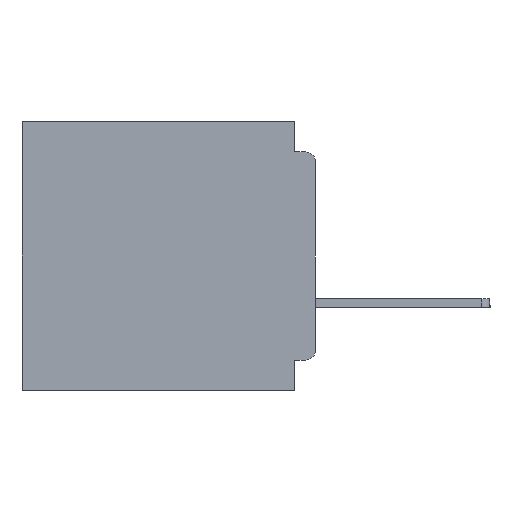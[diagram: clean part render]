
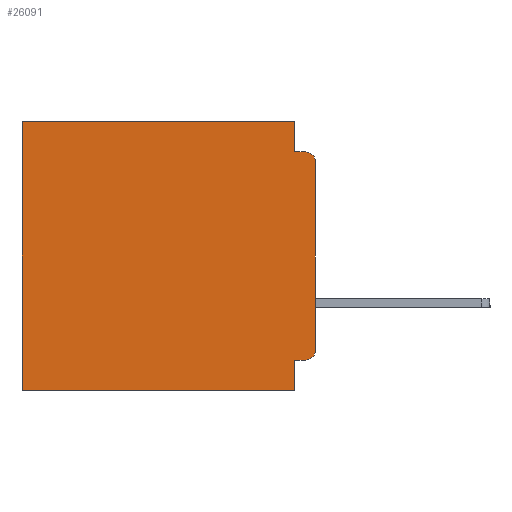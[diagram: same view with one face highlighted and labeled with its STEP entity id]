
A CAD part, left-side view. The second image highlights one B-rep face of the part: STEP entity #26091.
In plain terms, the highlighted planar face has unit normal (-1, 0, 0).
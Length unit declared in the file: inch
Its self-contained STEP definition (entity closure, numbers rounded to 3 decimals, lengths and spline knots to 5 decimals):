
#51 = DIRECTION ( 'NONE',  ( -1., 0., 0. ) ) ;
#653 = CARTESIAN_POINT ( 'NONE',  ( 0.3, 0., -0.34 ) ) ;
#697 = EDGE_CURVE ( 'NONE', #22691, #24776, #6762, .T. ) ;
#934 = EDGE_CURVE ( 'NONE', #24162, #24214, #21215, .T. ) ;
#1195 = VECTOR ( 'NONE', #26522, 39.37008 ) ;
#1617 = ORIENTED_EDGE ( 'NONE', *, *, #15779, .T. ) ;
#2592 = VERTEX_POINT ( 'NONE', #31737 ) ;
#3250 = CARTESIAN_POINT ( 'NONE',  ( 0.3, 0., -0.06 ) ) ;
#3530 = DIRECTION ( 'NONE',  ( 0., 0., -1. ) ) ;
#3794 = LINE ( 'NONE', #26457, #24612 ) ;
#4449 = VERTEX_POINT ( 'NONE', #22571 ) ;
#4848 = CARTESIAN_POINT ( 'NONE',  ( 0.3, 0.031, 0. ) ) ;
#5273 = VECTOR ( 'NONE', #8949, 39.37008 ) ;
#6329 = PLANE ( 'NONE',  #8413 ) ;
#6762 = LINE ( 'NONE', #13682, #28428 ) ;
#6907 = EDGE_CURVE ( 'NONE', #15076, #2592, #25308, .T. ) ;
#6944 = DIRECTION ( 'NONE',  ( 0., 0., -1. ) ) ;
#7821 = VECTOR ( 'NONE', #6944, 39.37008 ) ;
#8090 = CARTESIAN_POINT ( 'NONE',  ( 0.3, 0.015, -0.06 ) ) ;
#8413 = AXIS2_PLACEMENT_3D ( 'NONE', #26077, #12065, #31783 ) ;
#8621 = CARTESIAN_POINT ( 'NONE',  ( 0.3, 0., -0.4 ) ) ;
#8702 = LINE ( 'NONE', #23894, #7821 ) ;
#8949 = DIRECTION ( 'NONE',  ( 0., 0., -1. ) ) ;
#9824 = EDGE_CURVE ( 'NONE', #32559, #15076, #35727, .T. ) ;
#9935 = EDGE_CURVE ( 'NONE', #4449, #2592, #23817, .T. ) ;
#10116 = VECTOR ( 'NONE', #22009, 39.37008 ) ;
#10307 = VECTOR ( 'NONE', #26129, 39.37008 ) ;
#10469 = AXIS2_PLACEMENT_3D ( 'NONE', #8090, #27848, #10963 ) ;
#10963 = DIRECTION ( 'NONE',  ( 0., 0., -1. ) ) ;
#12027 = CARTESIAN_POINT ( 'NONE',  ( 0.3, 0.031, -0.4 ) ) ;
#12065 = DIRECTION ( 'NONE',  ( 1., 0., 0. ) ) ;
#12370 = VECTOR ( 'NONE', #3530, 39.37008 ) ;
#13682 = CARTESIAN_POINT ( 'NONE',  ( 0.3, 0., -0.045 ) ) ;
#14464 = CIRCLE ( 'NONE', #31461, 0.015 ) ;
#14805 = DIRECTION ( 'NONE',  ( 0., -1., 0. ) ) ;
#14817 = EDGE_CURVE ( 'NONE', #35808, #4449, #3794, .T. ) ;
#14842 = EDGE_CURVE ( 'NONE', #35808, #22691, #8702, .T. ) ;
#15076 = VERTEX_POINT ( 'NONE', #33397 ) ;
#15779 = EDGE_CURVE ( 'NONE', #23216, #24214, #14464, .T. ) ;
#17085 = CARTESIAN_POINT ( 'NONE',  ( 0.3, 0.015, -0.34 ) ) ;
#17675 = LINE ( 'NONE', #36063, #10116 ) ;
#18830 = EDGE_CURVE ( 'NONE', #24162, #24776, #29590, .T. ) ;
#19890 = DIRECTION ( 'NONE',  ( 0., 0., -1. ) ) ;
#21215 = LINE ( 'NONE', #8621, #5273 ) ;
#22009 = DIRECTION ( 'NONE',  ( 0., 1., 0. ) ) ;
#22571 = CARTESIAN_POINT ( 'NONE',  ( 0.3, 0.437, 0. ) ) ;
#22691 = VERTEX_POINT ( 'NONE', #30205 ) ;
#23216 = VERTEX_POINT ( 'NONE', #35714 ) ;
#23716 = CARTESIAN_POINT ( 'NONE',  ( 0.3, 0.437, -0.4 ) ) ;
#23817 = LINE ( 'NONE', #23716, #1195 ) ;
#23894 = CARTESIAN_POINT ( 'NONE',  ( 0.3, 0.031, 0. ) ) ;
#23969 = FACE_OUTER_BOUND ( 'NONE', #33503, .T. ) ;
#24162 = VERTEX_POINT ( 'NONE', #3250 ) ;
#24214 = VERTEX_POINT ( 'NONE', #653 ) ;
#24612 = VECTOR ( 'NONE', #35001, 39.37008 ) ;
#24776 = VERTEX_POINT ( 'NONE', #28713 ) ;
#25308 = LINE ( 'NONE', #28987, #10307 ) ;
#26077 = CARTESIAN_POINT ( 'NONE',  ( 0.3, 0., -0.4 ) ) ;
#26091 = ADVANCED_FACE ( 'NONE', ( #23969 ), #6329, .F. ) ;
#26129 = DIRECTION ( 'NONE',  ( 0., 1., 0. ) ) ;
#26457 = CARTESIAN_POINT ( 'NONE',  ( 0.3, 0., 0. ) ) ;
#26522 = DIRECTION ( 'NONE',  ( 0., 0., -1. ) ) ;
#27848 = DIRECTION ( 'NONE',  ( -1., 0., 0. ) ) ;
#28428 = VECTOR ( 'NONE', #14805, 39.37008 ) ;
#28656 = EDGE_CURVE ( 'NONE', #23216, #32559, #17675, .T. ) ;
#28713 = CARTESIAN_POINT ( 'NONE',  ( 0.3, 0.015, -0.045 ) ) ;
#28987 = CARTESIAN_POINT ( 'NONE',  ( 0.3, 0., -0.4 ) ) ;
#29137 = ORIENTED_EDGE ( 'NONE', *, *, #9935, .T. ) ;
#29404 = ORIENTED_EDGE ( 'NONE', *, *, #14817, .T. ) ;
#29590 = CIRCLE ( 'NONE', #10469, 0.015 ) ;
#30137 = ORIENTED_EDGE ( 'NONE', *, *, #14842, .F. ) ;
#30205 = CARTESIAN_POINT ( 'NONE',  ( 0.3, 0.031, -0.045 ) ) ;
#30388 = CARTESIAN_POINT ( 'NONE',  ( 0.3, 0.031, -0.355 ) ) ;
#30987 = ORIENTED_EDGE ( 'NONE', *, *, #697, .F. ) ;
#31461 = AXIS2_PLACEMENT_3D ( 'NONE', #17085, #51, #19890 ) ;
#31523 = ORIENTED_EDGE ( 'NONE', *, *, #18830, .T. ) ;
#31737 = CARTESIAN_POINT ( 'NONE',  ( 0.3, 0.437, -0.4 ) ) ;
#31783 = DIRECTION ( 'NONE',  ( 0., 0., -1. ) ) ;
#32193 = ORIENTED_EDGE ( 'NONE', *, *, #934, .F. ) ;
#32559 = VERTEX_POINT ( 'NONE', #30388 ) ;
#33397 = CARTESIAN_POINT ( 'NONE',  ( 0.3, 0.031, -0.4 ) ) ;
#33503 = EDGE_LOOP ( 'NONE', ( #32193, #31523, #30987, #30137, #29404, #29137, #34035, #33529, #34473, #1617 ) ) ;
#33529 = ORIENTED_EDGE ( 'NONE', *, *, #9824, .F. ) ;
#34035 = ORIENTED_EDGE ( 'NONE', *, *, #6907, .F. ) ;
#34473 = ORIENTED_EDGE ( 'NONE', *, *, #28656, .F. ) ;
#35001 = DIRECTION ( 'NONE',  ( 0., 1., 0. ) ) ;
#35714 = CARTESIAN_POINT ( 'NONE',  ( 0.3, 0.015, -0.355 ) ) ;
#35727 = LINE ( 'NONE', #12027, #12370 ) ;
#35808 = VERTEX_POINT ( 'NONE', #4848 ) ;
#36063 = CARTESIAN_POINT ( 'NONE',  ( 0.3, 0., -0.355 ) ) ;
